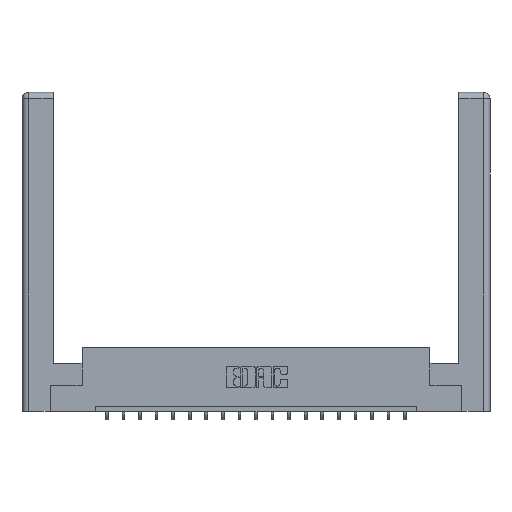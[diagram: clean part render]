
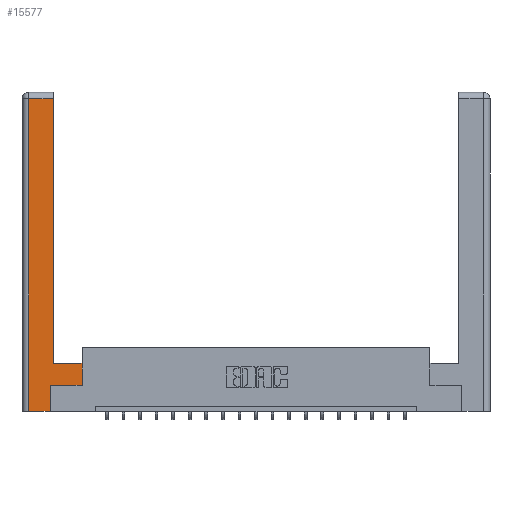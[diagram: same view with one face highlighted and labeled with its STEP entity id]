
A CAD part, top view. The second image highlights one B-rep face of the part: STEP entity #15577.
In plain terms, the highlighted planar face has unit normal (0, 0, 1).
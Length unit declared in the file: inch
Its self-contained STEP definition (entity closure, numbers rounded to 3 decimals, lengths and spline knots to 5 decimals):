
#157 = EDGE_CURVE ( 'NONE', #11082, #14409, #9247, .T. ) ;
#158 = LINE ( 'NONE', #14372, #15964 ) ;
#259 = ORIENTED_EDGE ( 'NONE', *, *, #8098, .T. ) ;
#435 = VERTEX_POINT ( 'NONE', #2425 ) ;
#493 = VERTEX_POINT ( 'NONE', #4062 ) ;
#832 = ORIENTED_EDGE ( 'NONE', *, *, #964, .T. ) ;
#949 = DIRECTION ( 'NONE',  ( 1., 0., 0. ) ) ;
#964 = EDGE_CURVE ( 'NONE', #435, #493, #158, .T. ) ;
#1352 = EDGE_CURVE ( 'NONE', #1968, #18108, #8021, .T. ) ;
#1968 = VERTEX_POINT ( 'NONE', #10666 ) ;
#2180 = EDGE_CURVE ( 'NONE', #14409, #1968, #12046, .T. ) ;
#2224 = DIRECTION ( 'NONE',  ( -1., 0., 0. ) ) ;
#2425 = CARTESIAN_POINT ( 'NONE',  ( 0.565, 0.45, 0. ) ) ;
#2722 = EDGE_LOOP ( 'NONE', ( #6472, #16458, #12391, #10996, #10868, #259, #12341, #832 ) ) ;
#3486 = VECTOR ( 'NONE', #5292, 39.37008 ) ;
#3962 = LINE ( 'NONE', #12789, #3486 ) ;
#4062 = CARTESIAN_POINT ( 'NONE',  ( 0.295, 0.45, 0. ) ) ;
#4507 = EDGE_CURVE ( 'NONE', #18108, #8512, #6463, .T. ) ;
#5292 = DIRECTION ( 'NONE',  ( 0., 1., 0. ) ) ;
#5369 = VECTOR ( 'NONE', #8368, 39.37008 ) ;
#6182 = DIRECTION ( 'NONE',  ( -1., 0., 0. ) ) ;
#6463 = LINE ( 'NONE', #14297, #10223 ) ;
#6472 = ORIENTED_EDGE ( 'NONE', *, *, #10678, .T. ) ;
#6675 = DIRECTION ( 'NONE',  ( 0., 1., 0. ) ) ;
#7043 = LINE ( 'NONE', #19136, #5369 ) ;
#7230 = CARTESIAN_POINT ( 'NONE',  ( 0.265, 0., 0. ) ) ;
#7270 = VECTOR ( 'NONE', #14236, 39.37008 ) ;
#7538 = VECTOR ( 'NONE', #949, 39.37008 ) ;
#8021 = LINE ( 'NONE', #7230, #7538 ) ;
#8098 = EDGE_CURVE ( 'NONE', #8512, #11084, #18571, .T. ) ;
#8346 = DIRECTION ( 'NONE',  ( 1., 0., 0. ) ) ;
#8368 = DIRECTION ( 'NONE',  ( 0., 1., 0. ) ) ;
#8512 = VERTEX_POINT ( 'NONE', #11908 ) ;
#9247 = LINE ( 'NONE', #10698, #11647 ) ;
#10223 = VECTOR ( 'NONE', #6675, 39.37008 ) ;
#10583 = EDGE_CURVE ( 'NONE', #11084, #435, #3962, .T. ) ;
#10666 = CARTESIAN_POINT ( 'NONE',  ( 0.0615, 0., 0. ) ) ;
#10678 = EDGE_CURVE ( 'NONE', #493, #11082, #7043, .T. ) ;
#10698 = CARTESIAN_POINT ( 'NONE',  ( 0.0615, 2.94, 0. ) ) ;
#10868 = ORIENTED_EDGE ( 'NONE', *, *, #4507, .T. ) ;
#10996 = ORIENTED_EDGE ( 'NONE', *, *, #1352, .T. ) ;
#11082 = VERTEX_POINT ( 'NONE', #17203 ) ;
#11084 = VERTEX_POINT ( 'NONE', #14383 ) ;
#11193 = AXIS2_PLACEMENT_3D ( 'NONE', #11353, #14252, #2224 ) ;
#11353 = CARTESIAN_POINT ( 'NONE',  ( 0., 0., 0. ) ) ;
#11647 = VECTOR ( 'NONE', #6182, 39.37008 ) ;
#11908 = CARTESIAN_POINT ( 'NONE',  ( 0.265, 0.245, 0. ) ) ;
#12046 = LINE ( 'NONE', #12619, #7270 ) ;
#12341 = ORIENTED_EDGE ( 'NONE', *, *, #10583, .T. ) ;
#12391 = ORIENTED_EDGE ( 'NONE', *, *, #2180, .T. ) ;
#12619 = CARTESIAN_POINT ( 'NONE',  ( 0.0615, 0., 0. ) ) ;
#12789 = CARTESIAN_POINT ( 'NONE',  ( 0.565, 0.45, 0. ) ) ;
#13913 = CARTESIAN_POINT ( 'NONE',  ( 0.265, 0., 0. ) ) ;
#14236 = DIRECTION ( 'NONE',  ( 0., -1., 0. ) ) ;
#14252 = DIRECTION ( 'NONE',  ( 0., 0., -1. ) ) ;
#14297 = CARTESIAN_POINT ( 'NONE',  ( 0.265, 0.245, 0. ) ) ;
#14372 = CARTESIAN_POINT ( 'NONE',  ( 0.295, 0.45, 0. ) ) ;
#14383 = CARTESIAN_POINT ( 'NONE',  ( 0.565, 0.245, 0. ) ) ;
#14409 = VERTEX_POINT ( 'NONE', #17178 ) ;
#15577 = ADVANCED_FACE ( 'NONE', ( #16354 ), #17265, .F. ) ;
#15964 = VECTOR ( 'NONE', #15976, 39.37008 ) ;
#15976 = DIRECTION ( 'NONE',  ( -1., 0., 0. ) ) ;
#16354 = FACE_OUTER_BOUND ( 'NONE', #2722, .T. ) ;
#16458 = ORIENTED_EDGE ( 'NONE', *, *, #157, .T. ) ;
#17147 = VECTOR ( 'NONE', #8346, 39.37008 ) ;
#17178 = CARTESIAN_POINT ( 'NONE',  ( 0.0615, 2.94, 0. ) ) ;
#17203 = CARTESIAN_POINT ( 'NONE',  ( 0.295, 2.94, 0. ) ) ;
#17265 = PLANE ( 'NONE',  #11193 ) ;
#18108 = VERTEX_POINT ( 'NONE', #13913 ) ;
#18571 = LINE ( 'NONE', #18806, #17147 ) ;
#18806 = CARTESIAN_POINT ( 'NONE',  ( 0.565, 0.245, 0. ) ) ;
#19136 = CARTESIAN_POINT ( 'NONE',  ( 0.295, 3., 0. ) ) ;
